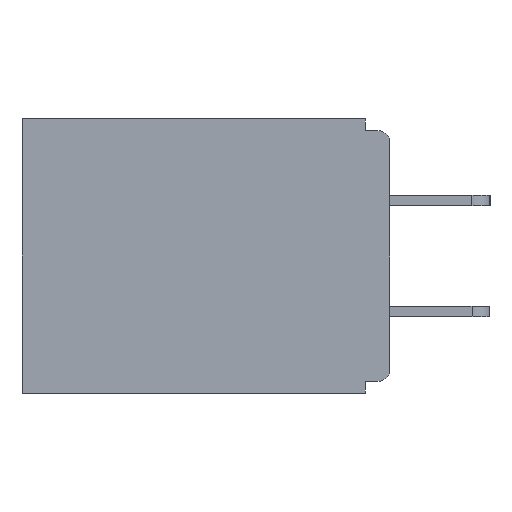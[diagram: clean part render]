
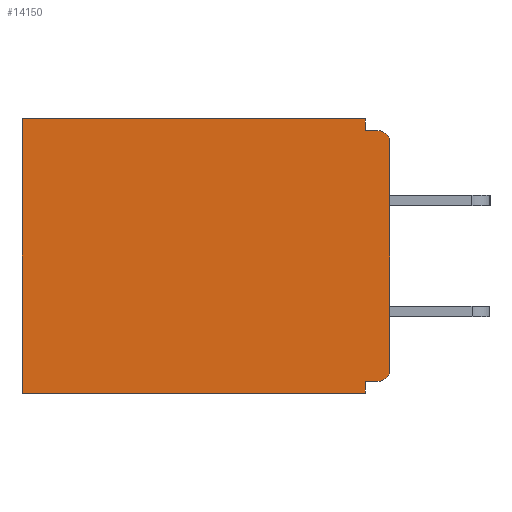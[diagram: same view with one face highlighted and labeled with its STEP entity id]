
A CAD part, left-side view. The second image highlights one B-rep face of the part: STEP entity #14150.
In plain terms, the highlighted planar face has unit normal (-1, 0, 0).
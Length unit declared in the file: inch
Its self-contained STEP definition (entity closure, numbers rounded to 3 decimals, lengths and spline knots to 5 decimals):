
#189 = CARTESIAN_POINT ( 'NONE',  ( 0.298, 0.031, -0.343 ) ) ;
#629 = VECTOR ( 'NONE', #17034, 39.37008 ) ;
#792 = VERTEX_POINT ( 'NONE', #22100 ) ;
#817 = DIRECTION ( 'NONE',  ( 0., 0., -1. ) ) ;
#1461 = AXIS2_PLACEMENT_3D ( 'NONE', #22183, #24498, #20152 ) ;
#1606 = AXIS2_PLACEMENT_3D ( 'NONE', #19813, #26903, #15184 ) ;
#1871 = VERTEX_POINT ( 'NONE', #13246 ) ;
#2964 = CARTESIAN_POINT ( 'NONE',  ( 0.298, 0., -0.328 ) ) ;
#3053 = VERTEX_POINT ( 'NONE', #14103 ) ;
#3109 = DIRECTION ( 'NONE',  ( 0., 1., 0. ) ) ;
#3389 = DIRECTION ( 'NONE',  ( 0., -1., 0. ) ) ;
#3989 = EDGE_CURVE ( 'NONE', #792, #28104, #5877, .T. ) ;
#4246 = VECTOR ( 'NONE', #3389, 39.37008 ) ;
#4718 = CARTESIAN_POINT ( 'NONE',  ( 0.298, 0.46, -0.343 ) ) ;
#4721 = EDGE_CURVE ( 'NONE', #25406, #21882, #27362, .T. ) ;
#4952 = LINE ( 'NONE', #17112, #4246 ) ;
#5105 = CARTESIAN_POINT ( 'NONE',  ( 0.298, 0.031, -0.328 ) ) ;
#5877 = LINE ( 'NONE', #7924, #19885 ) ;
#7317 = EDGE_CURVE ( 'NONE', #25406, #22338, #19125, .T. ) ;
#7519 = FACE_OUTER_BOUND ( 'NONE', #7562, .T. ) ;
#7562 = EDGE_LOOP ( 'NONE', ( #17878, #23298, #19202, #26788, #28892, #25090, #14556, #8447, #19690, #20276 ) ) ;
#7924 = CARTESIAN_POINT ( 'NONE',  ( 0.298, 0., 0. ) ) ;
#8447 = ORIENTED_EDGE ( 'NONE', *, *, #7317, .F. ) ;
#8603 = PLANE ( 'NONE',  #1461 ) ;
#9126 = DIRECTION ( 'NONE',  ( 0., 0., -1. ) ) ;
#9678 = DIRECTION ( 'NONE',  ( 0., 1., 0. ) ) ;
#9707 = LINE ( 'NONE', #20879, #19753 ) ;
#9878 = EDGE_CURVE ( 'NONE', #792, #23455, #9707, .T. ) ;
#9954 = CARTESIAN_POINT ( 'NONE',  ( 0.298, 0.015, -0.03 ) ) ;
#11054 = EDGE_CURVE ( 'NONE', #26923, #24421, #25455, .T. ) ;
#11701 = DIRECTION ( 'NONE',  ( 0., 0., -1. ) ) ;
#12214 = CARTESIAN_POINT ( 'NONE',  ( 0.298, 0., -0.343 ) ) ;
#12224 = DIRECTION ( 'NONE',  ( 0., 1., 0. ) ) ;
#12485 = CARTESIAN_POINT ( 'NONE',  ( 0.298, 0.46, 0. ) ) ;
#13246 = CARTESIAN_POINT ( 'NONE',  ( 0.298, 0.015, -0.015 ) ) ;
#13665 = DIRECTION ( 'NONE',  ( 0., 0., -1. ) ) ;
#14103 = CARTESIAN_POINT ( 'NONE',  ( 0.298, 0., -0.03 ) ) ;
#14150 = ADVANCED_FACE ( 'NONE', ( #7519 ), #8603, .F. ) ;
#14556 = ORIENTED_EDGE ( 'NONE', *, *, #26905, .F. ) ;
#14972 = EDGE_CURVE ( 'NONE', #3053, #21882, #17524, .T. ) ;
#15184 = DIRECTION ( 'NONE',  ( 0., 0., -1. ) ) ;
#15897 = VECTOR ( 'NONE', #9678, 39.37008 ) ;
#15947 = CARTESIAN_POINT ( 'NONE',  ( 0.298, 0.031, -0.343 ) ) ;
#16035 = EDGE_CURVE ( 'NONE', #23455, #1871, #4952, .T. ) ;
#17034 = DIRECTION ( 'NONE',  ( 0., 0., -1. ) ) ;
#17112 = CARTESIAN_POINT ( 'NONE',  ( 0.298, 0., -0.015 ) ) ;
#17524 = LINE ( 'NONE', #24096, #629 ) ;
#17878 = ORIENTED_EDGE ( 'NONE', *, *, #18655, .T. ) ;
#18655 = EDGE_CURVE ( 'NONE', #3053, #1871, #24548, .T. ) ;
#18801 = AXIS2_PLACEMENT_3D ( 'NONE', #9954, #26009, #817 ) ;
#19081 = CARTESIAN_POINT ( 'NONE',  ( 0.298, 0.031, -0.015 ) ) ;
#19125 = LINE ( 'NONE', #2964, #15897 ) ;
#19202 = ORIENTED_EDGE ( 'NONE', *, *, #9878, .F. ) ;
#19690 = ORIENTED_EDGE ( 'NONE', *, *, #4721, .T. ) ;
#19723 = CARTESIAN_POINT ( 'NONE',  ( 0.298, 0.015, -0.328 ) ) ;
#19753 = VECTOR ( 'NONE', #11701, 39.37008 ) ;
#19813 = CARTESIAN_POINT ( 'NONE',  ( 0.298, 0.015, -0.313 ) ) ;
#19885 = VECTOR ( 'NONE', #12224, 39.37008 ) ;
#20015 = VECTOR ( 'NONE', #9126, 39.37008 ) ;
#20152 = DIRECTION ( 'NONE',  ( 0., 0., -1. ) ) ;
#20276 = ORIENTED_EDGE ( 'NONE', *, *, #14972, .F. ) ;
#20356 = LINE ( 'NONE', #15947, #20015 ) ;
#20402 = VECTOR ( 'NONE', #3109, 39.37008 ) ;
#20879 = CARTESIAN_POINT ( 'NONE',  ( 0.298, 0.031, -0.343 ) ) ;
#21882 = VERTEX_POINT ( 'NONE', #22450 ) ;
#22100 = CARTESIAN_POINT ( 'NONE',  ( 0.298, 0.031, 0. ) ) ;
#22183 = CARTESIAN_POINT ( 'NONE',  ( 0.298, 0., 0. ) ) ;
#22338 = VERTEX_POINT ( 'NONE', #5105 ) ;
#22450 = CARTESIAN_POINT ( 'NONE',  ( 0.298, 0., -0.313 ) ) ;
#23298 = ORIENTED_EDGE ( 'NONE', *, *, #16035, .F. ) ;
#23455 = VERTEX_POINT ( 'NONE', #19081 ) ;
#23624 = LINE ( 'NONE', #27295, #28233 ) ;
#24096 = CARTESIAN_POINT ( 'NONE',  ( 0.298, 0., 0. ) ) ;
#24421 = VERTEX_POINT ( 'NONE', #4718 ) ;
#24498 = DIRECTION ( 'NONE',  ( 1., 0., 0. ) ) ;
#24548 = CIRCLE ( 'NONE', #18801, 0.015 ) ;
#25090 = ORIENTED_EDGE ( 'NONE', *, *, #11054, .F. ) ;
#25406 = VERTEX_POINT ( 'NONE', #19723 ) ;
#25455 = LINE ( 'NONE', #12214, #20402 ) ;
#26009 = DIRECTION ( 'NONE',  ( -1., 0., 0. ) ) ;
#26493 = EDGE_CURVE ( 'NONE', #28104, #24421, #23624, .T. ) ;
#26788 = ORIENTED_EDGE ( 'NONE', *, *, #3989, .T. ) ;
#26903 = DIRECTION ( 'NONE',  ( -1., 0., 0. ) ) ;
#26905 = EDGE_CURVE ( 'NONE', #22338, #26923, #20356, .T. ) ;
#26923 = VERTEX_POINT ( 'NONE', #189 ) ;
#27295 = CARTESIAN_POINT ( 'NONE',  ( 0.298, 0.46, 0. ) ) ;
#27362 = CIRCLE ( 'NONE', #1606, 0.015 ) ;
#28104 = VERTEX_POINT ( 'NONE', #12485 ) ;
#28233 = VECTOR ( 'NONE', #13665, 39.37008 ) ;
#28892 = ORIENTED_EDGE ( 'NONE', *, *, #26493, .T. ) ;
